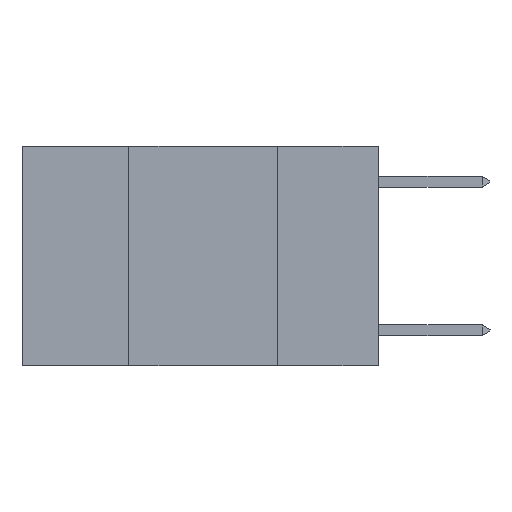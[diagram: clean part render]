
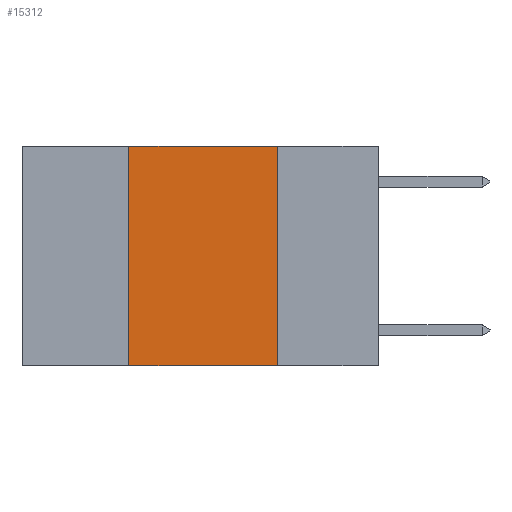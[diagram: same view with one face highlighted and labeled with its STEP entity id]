
A CAD part, left-side view. The second image highlights one B-rep face of the part: STEP entity #15312.
In plain terms, the highlighted planar face has unit normal (-1, 0, 0).
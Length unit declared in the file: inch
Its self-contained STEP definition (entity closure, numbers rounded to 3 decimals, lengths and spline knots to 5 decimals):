
#548 = LINE ( 'NONE', #8900, #8194 ) ;
#893 = DIRECTION ( 'NONE',  ( 0., -1., 0. ) ) ;
#1143 = EDGE_LOOP ( 'NONE', ( #17461, #17478, #17762, #17854 ) ) ;
#3552 = VERTEX_POINT ( 'NONE', #17521 ) ;
#3686 = AXIS2_PLACEMENT_3D ( 'NONE', #19731, #12228, #10787 ) ;
#5653 = VECTOR ( 'NONE', #7644, 39.37008 ) ;
#7644 = DIRECTION ( 'NONE',  ( 0., 0., 1. ) ) ;
#8194 = VECTOR ( 'NONE', #893, 39.37008 ) ;
#8794 = VERTEX_POINT ( 'NONE', #12260 ) ;
#8900 = CARTESIAN_POINT ( 'NONE',  ( 0., 0.6, 0. ) ) ;
#8922 = CARTESIAN_POINT ( 'NONE',  ( 0., 0.17, 0. ) ) ;
#10289 = CARTESIAN_POINT ( 'NONE',  ( 0., 0.42, 0. ) ) ;
#10787 = DIRECTION ( 'NONE',  ( 0., 0., -1. ) ) ;
#11923 = VECTOR ( 'NONE', #19411, 39.37008 ) ;
#12148 = LINE ( 'NONE', #15095, #18225 ) ;
#12228 = DIRECTION ( 'NONE',  ( 1., 0., 0. ) ) ;
#12260 = CARTESIAN_POINT ( 'NONE',  ( 0., 0.42, -0.37 ) ) ;
#12449 = EDGE_CURVE ( 'NONE', #15773, #3552, #548, .T. ) ;
#12610 = FACE_OUTER_BOUND ( 'NONE', #1143, .T. ) ;
#13662 = PLANE ( 'NONE',  #3686 ) ;
#14742 = EDGE_CURVE ( 'NONE', #8794, #18280, #12148, .T. ) ;
#15095 = CARTESIAN_POINT ( 'NONE',  ( 0., 0.6, -0.37 ) ) ;
#15153 = CARTESIAN_POINT ( 'NONE',  ( 0., 0.42, 0. ) ) ;
#15180 = EDGE_CURVE ( 'NONE', #3552, #18280, #18940, .T. ) ;
#15312 = ADVANCED_FACE ( 'NONE', ( #12610 ), #13662, .F. ) ;
#15773 = VERTEX_POINT ( 'NONE', #10289 ) ;
#15939 = CARTESIAN_POINT ( 'NONE',  ( 0., 0.17, -0.37 ) ) ;
#17461 = ORIENTED_EDGE ( 'NONE', *, *, #15180, .F. ) ;
#17478 = ORIENTED_EDGE ( 'NONE', *, *, #12449, .F. ) ;
#17521 = CARTESIAN_POINT ( 'NONE',  ( 0., 0.17, 0. ) ) ;
#17746 = LINE ( 'NONE', #15153, #5653 ) ;
#17762 = ORIENTED_EDGE ( 'NONE', *, *, #18556, .F. ) ;
#17854 = ORIENTED_EDGE ( 'NONE', *, *, #14742, .T. ) ;
#18225 = VECTOR ( 'NONE', #19616, 39.37008 ) ;
#18280 = VERTEX_POINT ( 'NONE', #15939 ) ;
#18556 = EDGE_CURVE ( 'NONE', #8794, #15773, #17746, .T. ) ;
#18940 = LINE ( 'NONE', #8922, #11923 ) ;
#19411 = DIRECTION ( 'NONE',  ( 0., 0., -1. ) ) ;
#19616 = DIRECTION ( 'NONE',  ( 0., -1., 0. ) ) ;
#19731 = CARTESIAN_POINT ( 'NONE',  ( 0., 0.6, 0. ) ) ;
